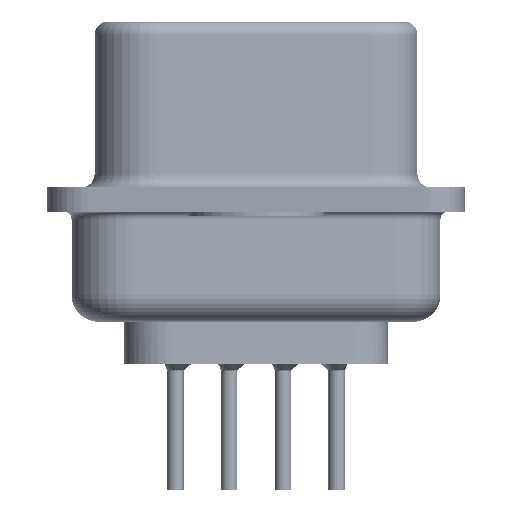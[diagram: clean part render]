
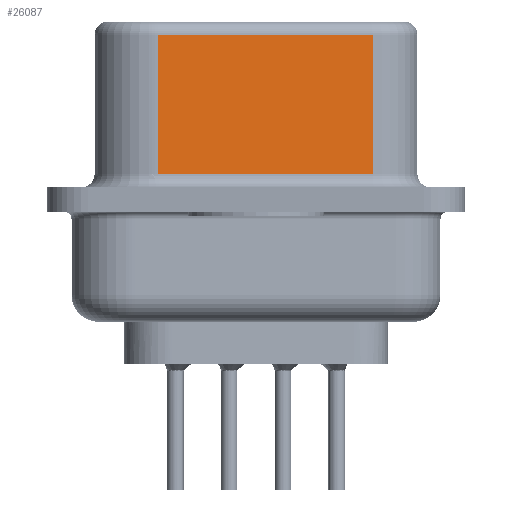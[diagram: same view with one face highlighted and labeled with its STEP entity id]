
A CAD part, left-side view. The second image highlights one B-rep face of the part: STEP entity #26087.
In plain terms, the highlighted planar face has unit normal (-0.985, -0.174, 0).
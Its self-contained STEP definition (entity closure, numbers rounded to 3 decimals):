
#74 = VECTOR ( 'NONE', #29465, 1000. ) ;
#285 = DIRECTION ( 'NONE',  ( 0.174, -0.985, 0. ) ) ;
#735 = VERTEX_POINT ( 'NONE', #31994 ) ;
#5240 = PLANE ( 'NONE',  #26699 ) ;
#5817 = DIRECTION ( 'NONE',  ( 0., 0., -1. ) ) ;
#7037 = CARTESIAN_POINT ( 'NONE',  ( 5.128, -4.297, 6.07 ) ) ;
#7598 = EDGE_CURVE ( 'NONE', #26111, #42039, #21434, .T. ) ;
#8337 = LINE ( 'NONE', #18798, #29456 ) ;
#12824 = ORIENTED_EDGE ( 'NONE', *, *, #7598, .T. ) ;
#15319 = EDGE_LOOP ( 'NONE', ( #20565, #33473, #30018, #12824 ) ) ;
#15548 = EDGE_CURVE ( 'NONE', #735, #26111, #15829, .T. ) ;
#15829 = LINE ( 'NONE', #36728, #74 ) ;
#17584 = CARTESIAN_POINT ( 'NONE',  ( 5.128, -4.297, 0.95 ) ) ;
#18798 = CARTESIAN_POINT ( 'NONE',  ( 5.128, -4.297, 6.57 ) ) ;
#18906 = DIRECTION ( 'NONE',  ( -0.174, 0.985, 0. ) ) ;
#20565 = ORIENTED_EDGE ( 'NONE', *, *, #24339, .F. ) ;
#20922 = LINE ( 'NONE', #7037, #29331 ) ;
#21434 = LINE ( 'NONE', #17584, #41459 ) ;
#22758 = CARTESIAN_POINT ( 'NONE',  ( 5.128, -4.297, 6.57 ) ) ;
#23045 = VERTEX_POINT ( 'NONE', #41421 ) ;
#24339 = EDGE_CURVE ( 'NONE', #23045, #42039, #8337, .T. ) ;
#25494 = CARTESIAN_POINT ( 'NONE',  ( 5.128, -4.297, 0.95 ) ) ;
#26087 = ADVANCED_FACE ( 'NONE', ( #36401 ), #5240, .F. ) ;
#26111 = VERTEX_POINT ( 'NONE', #40023 ) ;
#26699 = AXIS2_PLACEMENT_3D ( 'NONE', #22758, #39362, #18906 ) ;
#29331 = VECTOR ( 'NONE', #41821, 1000. ) ;
#29456 = VECTOR ( 'NONE', #5817, 1000. ) ;
#29465 = DIRECTION ( 'NONE',  ( 0., 0., -1. ) ) ;
#30018 = ORIENTED_EDGE ( 'NONE', *, *, #15548, .T. ) ;
#31994 = CARTESIAN_POINT ( 'NONE',  ( 3.735, 3.603, 6.07 ) ) ;
#33473 = ORIENTED_EDGE ( 'NONE', *, *, #39344, .T. ) ;
#36401 = FACE_OUTER_BOUND ( 'NONE', #15319, .T. ) ;
#36728 = CARTESIAN_POINT ( 'NONE',  ( 3.735, 3.603, 6.57 ) ) ;
#39344 = EDGE_CURVE ( 'NONE', #23045, #735, #20922, .T. ) ;
#39362 = DIRECTION ( 'NONE',  ( 0.985, 0.174, 0. ) ) ;
#40023 = CARTESIAN_POINT ( 'NONE',  ( 3.735, 3.603, 0.95 ) ) ;
#41421 = CARTESIAN_POINT ( 'NONE',  ( 5.128, -4.297, 6.07 ) ) ;
#41459 = VECTOR ( 'NONE', #285, 1000. ) ;
#41821 = DIRECTION ( 'NONE',  ( -0.174, 0.985, 0. ) ) ;
#42039 = VERTEX_POINT ( 'NONE', #25494 ) ;
